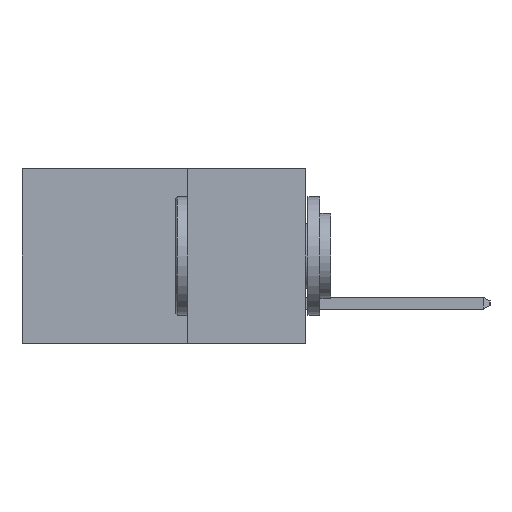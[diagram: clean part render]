
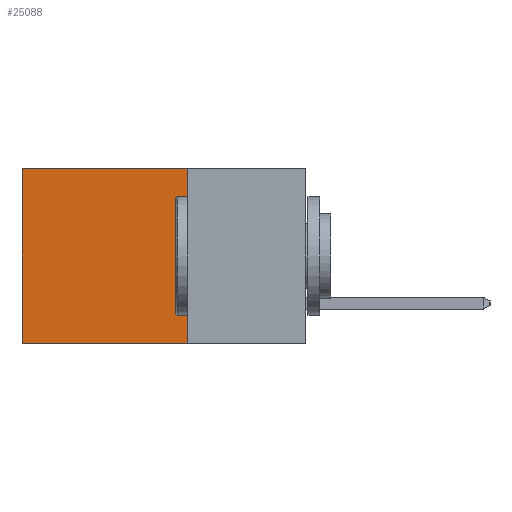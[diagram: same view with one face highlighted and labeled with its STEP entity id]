
A CAD part, left-side view. The second image highlights one B-rep face of the part: STEP entity #25088.
In plain terms, the highlighted planar face has unit normal (-1, 0, 0).
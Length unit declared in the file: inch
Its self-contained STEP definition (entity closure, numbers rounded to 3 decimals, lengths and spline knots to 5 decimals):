
#466 = EDGE_CURVE ( 'NONE', #9771, #18934, #22533, .T. ) ;
#882 = ORIENTED_EDGE ( 'NONE', *, *, #17327, .F. ) ;
#1695 = VECTOR ( 'NONE', #6305, 39.37008 ) ;
#2253 = EDGE_CURVE ( 'NONE', #18934, #3695, #10812, .T. ) ;
#3695 = VERTEX_POINT ( 'NONE', #19745 ) ;
#4301 = CARTESIAN_POINT ( 'NONE',  ( 0.298, 0.25, -0.37 ) ) ;
#5096 = CARTESIAN_POINT ( 'NONE',  ( 0.298, 0.25, 0. ) ) ;
#5746 = FACE_OUTER_BOUND ( 'NONE', #19376, .T. ) ;
#5777 = LINE ( 'NONE', #7823, #20627 ) ;
#6305 = DIRECTION ( 'NONE',  ( 0., 1., 0. ) ) ;
#6975 = LINE ( 'NONE', #4301, #1695 ) ;
#7103 = DIRECTION ( 'NONE',  ( 1., 0., 0. ) ) ;
#7558 = EDGE_CURVE ( 'NONE', #13373, #3695, #6975, .T. ) ;
#7823 = CARTESIAN_POINT ( 'NONE',  ( 0.298, 0.25, 0. ) ) ;
#9771 = VERTEX_POINT ( 'NONE', #17014 ) ;
#9796 = DIRECTION ( 'NONE',  ( 0., 0., -1. ) ) ;
#9986 = ORIENTED_EDGE ( 'NONE', *, *, #466, .T. ) ;
#10003 = CARTESIAN_POINT ( 'NONE',  ( 0.298, 0.6, 0. ) ) ;
#10065 = ORIENTED_EDGE ( 'NONE', *, *, #7558, .F. ) ;
#10375 = CARTESIAN_POINT ( 'NONE',  ( 0.298, 0.6, 0. ) ) ;
#10812 = LINE ( 'NONE', #10375, #14740 ) ;
#13373 = VERTEX_POINT ( 'NONE', #23814 ) ;
#14740 = VECTOR ( 'NONE', #22391, 39.37008 ) ;
#16778 = PLANE ( 'NONE',  #19326 ) ;
#17014 = CARTESIAN_POINT ( 'NONE',  ( 0.298, 0.25, 0. ) ) ;
#17327 = EDGE_CURVE ( 'NONE', #9771, #13373, #5777, .T. ) ;
#17508 = CARTESIAN_POINT ( 'NONE',  ( 0.298, 0.25, 0. ) ) ;
#17873 = DIRECTION ( 'NONE',  ( 0., 1., 0. ) ) ;
#18934 = VERTEX_POINT ( 'NONE', #10003 ) ;
#19326 = AXIS2_PLACEMENT_3D ( 'NONE', #5096, #7103, #20623 ) ;
#19376 = EDGE_LOOP ( 'NONE', ( #20929, #10065, #882, #9986 ) ) ;
#19745 = CARTESIAN_POINT ( 'NONE',  ( 0.298, 0.6, -0.37 ) ) ;
#20623 = DIRECTION ( 'NONE',  ( 0., 0., -1. ) ) ;
#20627 = VECTOR ( 'NONE', #9796, 39.37008 ) ;
#20929 = ORIENTED_EDGE ( 'NONE', *, *, #2253, .T. ) ;
#21927 = VECTOR ( 'NONE', #17873, 39.37008 ) ;
#22391 = DIRECTION ( 'NONE',  ( 0., 0., -1. ) ) ;
#22533 = LINE ( 'NONE', #17508, #21927 ) ;
#23814 = CARTESIAN_POINT ( 'NONE',  ( 0.298, 0.25, -0.37 ) ) ;
#25088 = ADVANCED_FACE ( 'NONE', ( #5746 ), #16778, .F. ) ;
